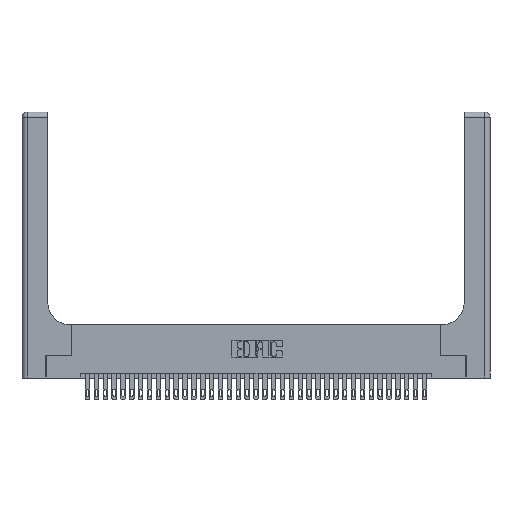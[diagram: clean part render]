
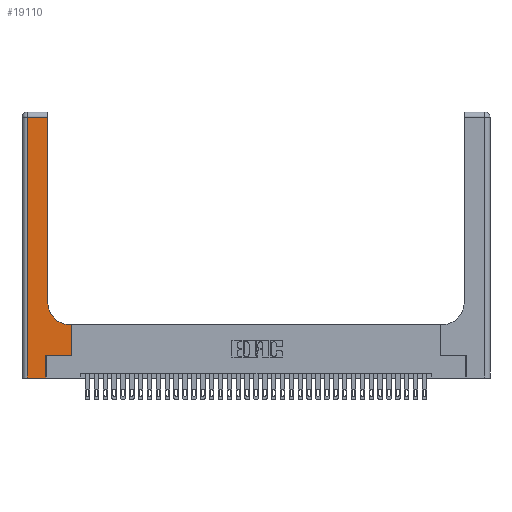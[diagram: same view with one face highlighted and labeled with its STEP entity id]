
A CAD part, top view. The second image highlights one B-rep face of the part: STEP entity #19110.
In plain terms, the highlighted planar face has unit normal (0, 0, 1).
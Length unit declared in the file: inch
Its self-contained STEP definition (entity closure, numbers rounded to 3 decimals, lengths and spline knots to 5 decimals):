
#254 = VERTEX_POINT ( 'NONE', #27150 ) ;
#1141 = EDGE_CURVE ( 'NONE', #20681, #11308, #29088, .T. ) ;
#2892 = VECTOR ( 'NONE', #14718, 39.37008 ) ;
#3401 = VECTOR ( 'NONE', #19617, 39.37008 ) ;
#3594 = LINE ( 'NONE', #35009, #32369 ) ;
#3830 = LINE ( 'NONE', #6013, #3401 ) ;
#4320 = VECTOR ( 'NONE', #28486, 39.37008 ) ;
#4475 = CARTESIAN_POINT ( 'NONE',  ( 0.269, 0., 0.37 ) ) ;
#4678 = EDGE_CURVE ( 'NONE', #20642, #28611, #13673, .T. ) ;
#4692 = EDGE_CURVE ( 'NONE', #27066, #20642, #3594, .T. ) ;
#5326 = LINE ( 'NONE', #17554, #22244 ) ;
#5358 = DIRECTION ( 'NONE',  ( 0., 0., -1. ) ) ;
#5371 = EDGE_LOOP ( 'NONE', ( #8231, #22113, #19993, #9872, #29052, #15832, #23500, #35470, #12596 ) ) ;
#5544 = LINE ( 'NONE', #26750, #26399 ) ;
#5801 = DIRECTION ( 'NONE',  ( 0., 0., -1. ) ) ;
#6013 = CARTESIAN_POINT ( 'NONE',  ( 0.06, 3., 0.37 ) ) ;
#6753 = FACE_OUTER_BOUND ( 'NONE', #5371, .T. ) ;
#8231 = ORIENTED_EDGE ( 'NONE', *, *, #15917, .T. ) ;
#8482 = LINE ( 'NONE', #13984, #11542 ) ;
#8580 = CARTESIAN_POINT ( 'NONE',  ( 0.5585, 0.6, 0.37 ) ) ;
#9872 = ORIENTED_EDGE ( 'NONE', *, *, #32795, .T. ) ;
#10582 = DIRECTION ( 'NONE',  ( 0., 1., 0. ) ) ;
#10776 = EDGE_CURVE ( 'NONE', #26658, #29643, #5544, .T. ) ;
#11308 = VERTEX_POINT ( 'NONE', #29125 ) ;
#11435 = CARTESIAN_POINT ( 'NONE',  ( 0.269, 0., 0.37 ) ) ;
#11542 = VECTOR ( 'NONE', #33478, 39.37008 ) ;
#11723 = CARTESIAN_POINT ( 'NONE',  ( 0.269, 0.25, 0.37 ) ) ;
#12422 = DIRECTION ( 'NONE',  ( -1., 0., 0. ) ) ;
#12596 = ORIENTED_EDGE ( 'NONE', *, *, #4678, .T. ) ;
#12798 = PLANE ( 'NONE',  #22370 ) ;
#13673 = CIRCLE ( 'NONE', #23735, 0.25 ) ;
#13984 = CARTESIAN_POINT ( 'NONE',  ( 0., 0., 0.37 ) ) ;
#14718 = DIRECTION ( 'NONE',  ( 0., 1., 0. ) ) ;
#15236 = DIRECTION ( 'NONE',  ( -1., 0., 0. ) ) ;
#15275 = DIRECTION ( 'NONE',  ( 0., 1., 0. ) ) ;
#15832 = ORIENTED_EDGE ( 'NONE', *, *, #1141, .T. ) ;
#15917 = EDGE_CURVE ( 'NONE', #28611, #26658, #5326, .T. ) ;
#17554 = CARTESIAN_POINT ( 'NONE',  ( 0.2915, 3., 0.37 ) ) ;
#18454 = EDGE_CURVE ( 'NONE', #11308, #27066, #20259, .T. ) ;
#19110 = ADVANCED_FACE ( 'NONE', ( #6753 ), #12798, .F. ) ;
#19617 = DIRECTION ( 'NONE',  ( 0., -1., 0. ) ) ;
#19886 = CARTESIAN_POINT ( 'NONE',  ( 0.5585, 0.25, 0.37 ) ) ;
#19993 = ORIENTED_EDGE ( 'NONE', *, *, #30800, .T. ) ;
#20259 = LINE ( 'NONE', #19886, #2892 ) ;
#20601 = LINE ( 'NONE', #4475, #32895 ) ;
#20642 = VERTEX_POINT ( 'NONE', #27221 ) ;
#20681 = VERTEX_POINT ( 'NONE', #32600 ) ;
#22113 = ORIENTED_EDGE ( 'NONE', *, *, #10776, .T. ) ;
#22244 = VECTOR ( 'NONE', #15275, 39.37008 ) ;
#22370 = AXIS2_PLACEMENT_3D ( 'NONE', #33139, #5358, #30044 ) ;
#23500 = ORIENTED_EDGE ( 'NONE', *, *, #18454, .T. ) ;
#23735 = AXIS2_PLACEMENT_3D ( 'NONE', #26644, #5801, #26054 ) ;
#26054 = DIRECTION ( 'NONE',  ( 1., 0., 0. ) ) ;
#26200 = CARTESIAN_POINT ( 'NONE',  ( 0.06, 2.94, 0.37 ) ) ;
#26399 = VECTOR ( 'NONE', #12422, 39.37008 ) ;
#26644 = CARTESIAN_POINT ( 'NONE',  ( 0.5415, 0.85, 0.37 ) ) ;
#26658 = VERTEX_POINT ( 'NONE', #29508 ) ;
#26732 = EDGE_CURVE ( 'NONE', #35258, #20681, #20601, .T. ) ;
#26750 = CARTESIAN_POINT ( 'NONE',  ( 0., 2.94, 0.37 ) ) ;
#27066 = VERTEX_POINT ( 'NONE', #8580 ) ;
#27150 = CARTESIAN_POINT ( 'NONE',  ( 0.06, 0., 0.37 ) ) ;
#27221 = CARTESIAN_POINT ( 'NONE',  ( 0.5415, 0.6, 0.37 ) ) ;
#28486 = DIRECTION ( 'NONE',  ( 1., 0., 0. ) ) ;
#28611 = VERTEX_POINT ( 'NONE', #34469 ) ;
#29052 = ORIENTED_EDGE ( 'NONE', *, *, #26732, .T. ) ;
#29088 = LINE ( 'NONE', #11723, #4320 ) ;
#29125 = CARTESIAN_POINT ( 'NONE',  ( 0.5585, 0.25, 0.37 ) ) ;
#29508 = CARTESIAN_POINT ( 'NONE',  ( 0.2915, 2.94, 0.37 ) ) ;
#29643 = VERTEX_POINT ( 'NONE', #26200 ) ;
#30044 = DIRECTION ( 'NONE',  ( -1., 0., 0. ) ) ;
#30800 = EDGE_CURVE ( 'NONE', #29643, #254, #3830, .T. ) ;
#32369 = VECTOR ( 'NONE', #15236, 39.37008 ) ;
#32600 = CARTESIAN_POINT ( 'NONE',  ( 0.269, 0.25, 0.37 ) ) ;
#32795 = EDGE_CURVE ( 'NONE', #254, #35258, #8482, .T. ) ;
#32895 = VECTOR ( 'NONE', #10582, 39.37008 ) ;
#33139 = CARTESIAN_POINT ( 'NONE',  ( 0., 3., 0.37 ) ) ;
#33478 = DIRECTION ( 'NONE',  ( 1., 0., 0. ) ) ;
#34469 = CARTESIAN_POINT ( 'NONE',  ( 0.2915, 0.85, 0.37 ) ) ;
#35009 = CARTESIAN_POINT ( 'NONE',  ( 0.2915, 0.6, 0.37 ) ) ;
#35258 = VERTEX_POINT ( 'NONE', #11435 ) ;
#35470 = ORIENTED_EDGE ( 'NONE', *, *, #4692, .T. ) ;
